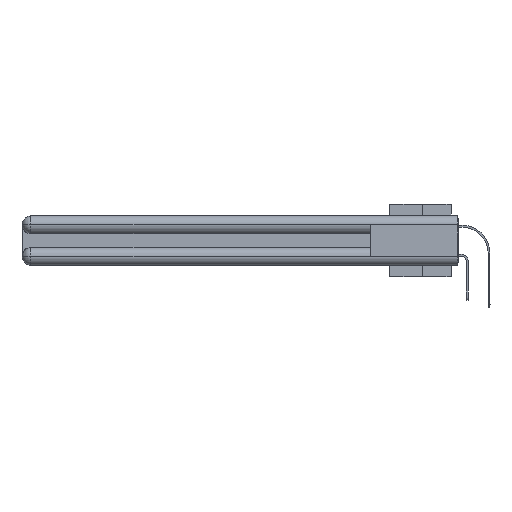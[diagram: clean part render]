
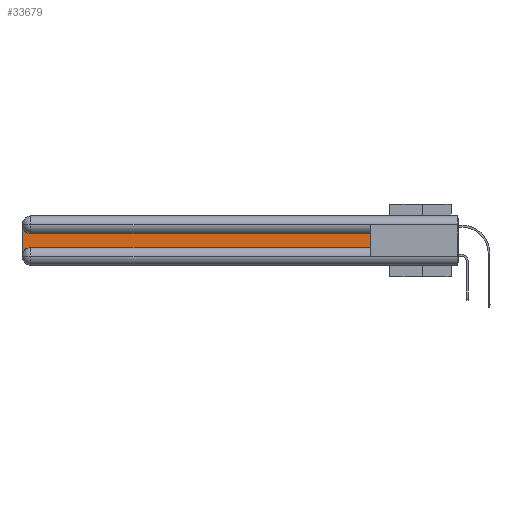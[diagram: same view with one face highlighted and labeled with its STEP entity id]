
A CAD part, left-side view. The second image highlights one B-rep face of the part: STEP entity #33679.
In plain terms, the highlighted planar face has unit normal (-1, 0, 0).
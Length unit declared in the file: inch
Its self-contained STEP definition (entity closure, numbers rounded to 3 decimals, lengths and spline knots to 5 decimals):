
#1103 = EDGE_CURVE ( 'NONE', #32221, #3996, #30251, .T. ) ;
#3271 = CARTESIAN_POINT ( 'NONE',  ( 0.075, 0.6, -0.2175 ) ) ;
#3498 = CARTESIAN_POINT ( 'NONE',  ( 0.075, 3., -0.0625 ) ) ;
#3577 = CARTESIAN_POINT ( 'NONE',  ( 0.075, 0.6, -0.1225 ) ) ;
#3996 = VERTEX_POINT ( 'NONE', #3498 ) ;
#6215 = DIRECTION ( 'NONE',  ( 0., -1., 0. ) ) ;
#6339 = CIRCLE ( 'NONE', #25084, 0.06 ) ;
#6357 = CARTESIAN_POINT ( 'NONE',  ( 0.075, 2.94, -0.1225 ) ) ;
#7209 = DIRECTION ( 'NONE',  ( 1., 0., 0. ) ) ;
#8296 = CARTESIAN_POINT ( 'NONE',  ( 0.075, 2.94, -0.0625 ) ) ;
#8872 = DIRECTION ( 'NONE',  ( 1., 0., 0. ) ) ;
#9399 = DIRECTION ( 'NONE',  ( 0., 0., -1. ) ) ;
#9647 = VERTEX_POINT ( 'NONE', #19938 ) ;
#10387 = ORIENTED_EDGE ( 'NONE', *, *, #19488, .T. ) ;
#12095 = VECTOR ( 'NONE', #22037, 39.37008 ) ;
#12545 = EDGE_CURVE ( 'NONE', #15146, #32221, #40779, .T. ) ;
#12959 = EDGE_CURVE ( 'NONE', #9647, #15146, #22380, .T. ) ;
#13472 = CARTESIAN_POINT ( 'NONE',  ( 0.075, 2.94, -0.2175 ) ) ;
#13515 = AXIS2_PLACEMENT_3D ( 'NONE', #8296, #21082, #33879 ) ;
#14320 = VERTEX_POINT ( 'NONE', #35965 ) ;
#15146 = VERTEX_POINT ( 'NONE', #3577 ) ;
#15725 = VECTOR ( 'NONE', #6215, 39.37008 ) ;
#16763 = VECTOR ( 'NONE', #9399, 39.37008 ) ;
#17914 = DIRECTION ( 'NONE',  ( 0., 1., 0. ) ) ;
#18079 = ORIENTED_EDGE ( 'NONE', *, *, #12545, .T. ) ;
#18599 = ORIENTED_EDGE ( 'NONE', *, *, #12959, .T. ) ;
#19237 = ORIENTED_EDGE ( 'NONE', *, *, #34710, .T. ) ;
#19488 = EDGE_CURVE ( 'NONE', #28220, #9647, #22772, .T. ) ;
#19938 = CARTESIAN_POINT ( 'NONE',  ( 0.075, 0.6, -0.2175 ) ) ;
#21028 = CARTESIAN_POINT ( 'NONE',  ( 0.075, 3., -0.1225 ) ) ;
#21082 = DIRECTION ( 'NONE',  ( 1., 0., 0. ) ) ;
#21577 = ORIENTED_EDGE ( 'NONE', *, *, #40973, .T. ) ;
#22037 = DIRECTION ( 'NONE',  ( 0., 0., 1. ) ) ;
#22380 = LINE ( 'NONE', #37932, #12095 ) ;
#22772 = LINE ( 'NONE', #3271, #15725 ) ;
#24207 = CARTESIAN_POINT ( 'NONE',  ( 0.075, 0.6, -0.1225 ) ) ;
#25084 = AXIS2_PLACEMENT_3D ( 'NONE', #39525, #7209, #32804 ) ;
#28220 = VERTEX_POINT ( 'NONE', #13472 ) ;
#28883 = LINE ( 'NONE', #38134, #16763 ) ;
#30251 = CIRCLE ( 'NONE', #13515, 0.06 ) ;
#30894 = FACE_OUTER_BOUND ( 'NONE', #35902, .T. ) ;
#32221 = VERTEX_POINT ( 'NONE', #6357 ) ;
#32804 = DIRECTION ( 'NONE',  ( 0., 0., -1. ) ) ;
#32851 = AXIS2_PLACEMENT_3D ( 'NONE', #21028, #8872, #41170 ) ;
#33679 = ADVANCED_FACE ( 'NONE', ( #30894 ), #34248, .F. ) ;
#33879 = DIRECTION ( 'NONE',  ( 0., 0., -1. ) ) ;
#34248 = PLANE ( 'NONE',  #32851 ) ;
#34257 = VECTOR ( 'NONE', #17914, 39.37008 ) ;
#34710 = EDGE_CURVE ( 'NONE', #3996, #14320, #28883, .T. ) ;
#35611 = ORIENTED_EDGE ( 'NONE', *, *, #1103, .T. ) ;
#35902 = EDGE_LOOP ( 'NONE', ( #18079, #35611, #19237, #21577, #10387, #18599 ) ) ;
#35965 = CARTESIAN_POINT ( 'NONE',  ( 0.075, 3., -0.2775 ) ) ;
#37932 = CARTESIAN_POINT ( 'NONE',  ( 0.075, 0.6, -0.2175 ) ) ;
#38134 = CARTESIAN_POINT ( 'NONE',  ( 0.075, 3., -0.2175 ) ) ;
#39525 = CARTESIAN_POINT ( 'NONE',  ( 0.075, 2.94, -0.2775 ) ) ;
#40779 = LINE ( 'NONE', #24207, #34257 ) ;
#40973 = EDGE_CURVE ( 'NONE', #14320, #28220, #6339, .T. ) ;
#41170 = DIRECTION ( 'NONE',  ( 0., 0., -1. ) ) ;
